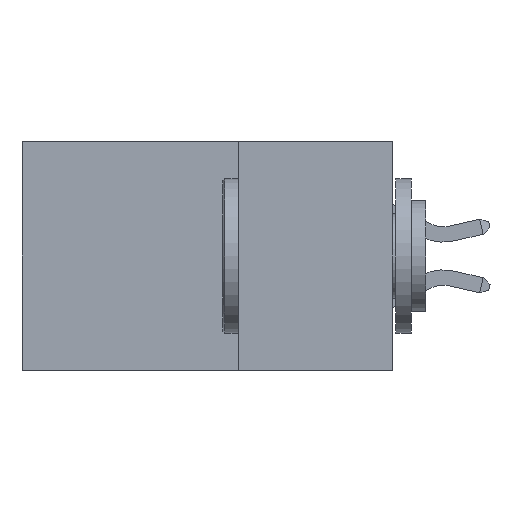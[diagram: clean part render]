
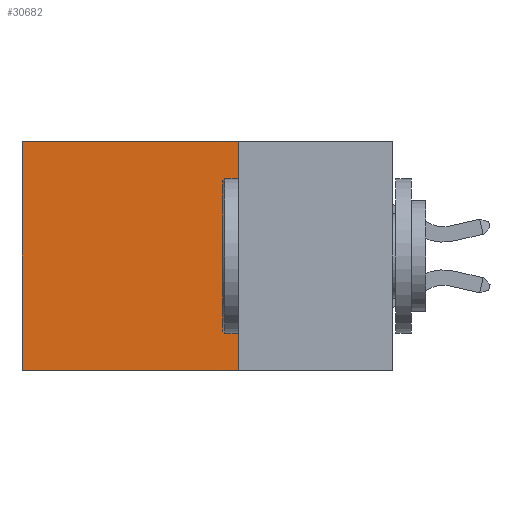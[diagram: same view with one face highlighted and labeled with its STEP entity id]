
A CAD part, left-side view. The second image highlights one B-rep face of the part: STEP entity #30682.
In plain terms, the highlighted planar face has unit normal (-1, 0, 0).
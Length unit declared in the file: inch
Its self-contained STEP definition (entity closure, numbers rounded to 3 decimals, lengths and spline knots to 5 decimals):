
#563 = AXIS2_PLACEMENT_3D ( 'NONE', #36494, #22961, #2836 ) ;
#806 = CARTESIAN_POINT ( 'NONE',  ( 0.2875, 0.25, 0. ) ) ;
#2836 = DIRECTION ( 'NONE',  ( 0., 0., -1. ) ) ;
#4472 = CARTESIAN_POINT ( 'NONE',  ( 0.2875, 0.6, 0. ) ) ;
#5178 = LINE ( 'NONE', #7874, #32549 ) ;
#6286 = CARTESIAN_POINT ( 'NONE',  ( 0.2875, 0.6, -0.37 ) ) ;
#7874 = CARTESIAN_POINT ( 'NONE',  ( 0.2875, 0.25, -0.37 ) ) ;
#8583 = DIRECTION ( 'NONE',  ( 0., 0., -1. ) ) ;
#8976 = DIRECTION ( 'NONE',  ( 0., 1., 0. ) ) ;
#9212 = VECTOR ( 'NONE', #8976, 39.37008 ) ;
#9351 = ORIENTED_EDGE ( 'NONE', *, *, #27546, .T. ) ;
#9466 = VERTEX_POINT ( 'NONE', #4472 ) ;
#9888 = PLANE ( 'NONE',  #563 ) ;
#12529 = EDGE_LOOP ( 'NONE', ( #23629, #34961, #26195, #9351 ) ) ;
#14491 = LINE ( 'NONE', #32369, #16614 ) ;
#14979 = CARTESIAN_POINT ( 'NONE',  ( 0.2875, 0.25, -0.37 ) ) ;
#15518 = VERTEX_POINT ( 'NONE', #806 ) ;
#16614 = VECTOR ( 'NONE', #8583, 39.37008 ) ;
#20945 = LINE ( 'NONE', #21382, #25198 ) ;
#21365 = VERTEX_POINT ( 'NONE', #6286 ) ;
#21382 = CARTESIAN_POINT ( 'NONE',  ( 0.2875, 0.6, 0. ) ) ;
#22326 = CARTESIAN_POINT ( 'NONE',  ( 0.2875, 0.25, 0. ) ) ;
#22961 = DIRECTION ( 'NONE',  ( 1., 0., 0. ) ) ;
#23629 = ORIENTED_EDGE ( 'NONE', *, *, #25268, .T. ) ;
#25198 = VECTOR ( 'NONE', #41076, 39.37008 ) ;
#25268 = EDGE_CURVE ( 'NONE', #9466, #21365, #20945, .T. ) ;
#25319 = EDGE_CURVE ( 'NONE', #33011, #21365, #5178, .T. ) ;
#26195 = ORIENTED_EDGE ( 'NONE', *, *, #35599, .F. ) ;
#27546 = EDGE_CURVE ( 'NONE', #15518, #9466, #29753, .T. ) ;
#28024 = DIRECTION ( 'NONE',  ( 0., 1., 0. ) ) ;
#29753 = LINE ( 'NONE', #22326, #9212 ) ;
#30682 = ADVANCED_FACE ( 'NONE', ( #35254 ), #9888, .F. ) ;
#32369 = CARTESIAN_POINT ( 'NONE',  ( 0.2875, 0.25, 0. ) ) ;
#32549 = VECTOR ( 'NONE', #28024, 39.37008 ) ;
#33011 = VERTEX_POINT ( 'NONE', #14979 ) ;
#34961 = ORIENTED_EDGE ( 'NONE', *, *, #25319, .F. ) ;
#35254 = FACE_OUTER_BOUND ( 'NONE', #12529, .T. ) ;
#35599 = EDGE_CURVE ( 'NONE', #15518, #33011, #14491, .T. ) ;
#36494 = CARTESIAN_POINT ( 'NONE',  ( 0.2875, 0.25, 0. ) ) ;
#41076 = DIRECTION ( 'NONE',  ( 0., 0., -1. ) ) ;
